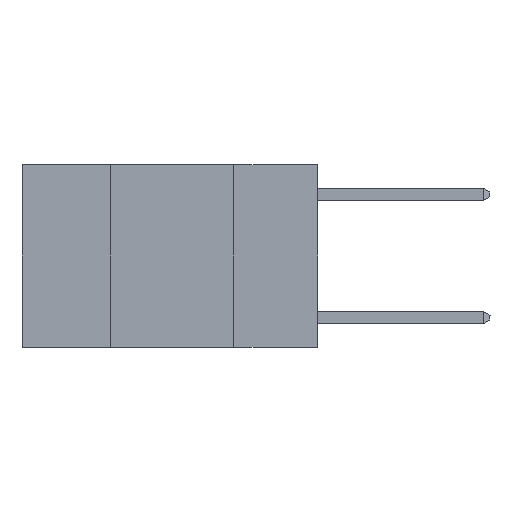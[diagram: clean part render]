
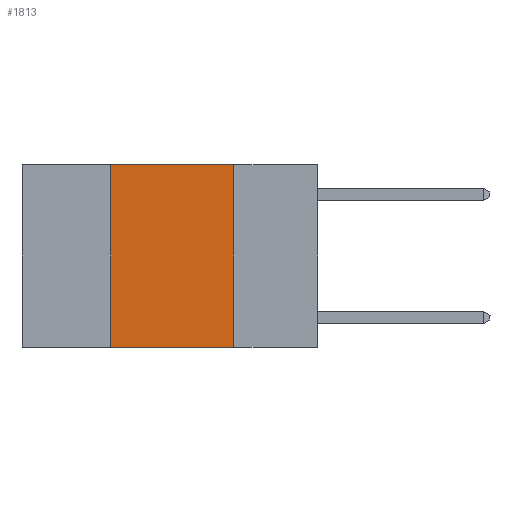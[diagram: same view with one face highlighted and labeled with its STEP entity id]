
A CAD part, left-side view. The second image highlights one B-rep face of the part: STEP entity #1813.
In plain terms, the highlighted planar face has unit normal (-1, 0, 0).
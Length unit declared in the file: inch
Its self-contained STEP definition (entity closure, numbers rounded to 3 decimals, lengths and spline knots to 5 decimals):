
#105 = CARTESIAN_POINT ( 'NONE',  ( 0., 0.6, 0. ) ) ;
#199 = EDGE_CURVE ( 'NONE', #4627, #4568, #7229, .T. ) ;
#1619 = DIRECTION ( 'NONE',  ( 0., -1., 0. ) ) ;
#1813 = ADVANCED_FACE ( 'NONE', ( #17642 ), #10746, .F. ) ;
#2471 = CARTESIAN_POINT ( 'NONE',  ( 0., 0.42, 0. ) ) ;
#3168 = DIRECTION ( 'NONE',  ( 0., -1., 0. ) ) ;
#3642 = DIRECTION ( 'NONE',  ( 0., 0., 1. ) ) ;
#4334 = CARTESIAN_POINT ( 'NONE',  ( 0., 0.42, -0.37 ) ) ;
#4423 = EDGE_CURVE ( 'NONE', #17658, #17810, #11080, .T. ) ;
#4512 = ORIENTED_EDGE ( 'NONE', *, *, #7670, .T. ) ;
#4556 = DIRECTION ( 'NONE',  ( 0., 0., -1. ) ) ;
#4568 = VERTEX_POINT ( 'NONE', #15377 ) ;
#4627 = VERTEX_POINT ( 'NONE', #8322 ) ;
#4974 = VECTOR ( 'NONE', #3642, 39.37008 ) ;
#5052 = DIRECTION ( 'NONE',  ( 0., 0., -1. ) ) ;
#5207 = ORIENTED_EDGE ( 'NONE', *, *, #199, .F. ) ;
#6779 = ORIENTED_EDGE ( 'NONE', *, *, #8624, .F. ) ;
#6850 = CARTESIAN_POINT ( 'NONE',  ( 0., 0.42, 0. ) ) ;
#7229 = LINE ( 'NONE', #10254, #7564 ) ;
#7535 = VECTOR ( 'NONE', #3168, 39.37008 ) ;
#7564 = VECTOR ( 'NONE', #4556, 39.37008 ) ;
#7670 = EDGE_CURVE ( 'NONE', #17658, #4568, #8884, .T. ) ;
#8236 = EDGE_LOOP ( 'NONE', ( #5207, #6779, #14369, #4512 ) ) ;
#8322 = CARTESIAN_POINT ( 'NONE',  ( 0., 0.17, 0. ) ) ;
#8599 = CARTESIAN_POINT ( 'NONE',  ( 0., 0.6, -0.37 ) ) ;
#8624 = EDGE_CURVE ( 'NONE', #17810, #4627, #16936, .T. ) ;
#8884 = LINE ( 'NONE', #8599, #14267 ) ;
#10254 = CARTESIAN_POINT ( 'NONE',  ( 0., 0.17, 0. ) ) ;
#10746 = PLANE ( 'NONE',  #10968 ) ;
#10968 = AXIS2_PLACEMENT_3D ( 'NONE', #13439, #14965, #5052 ) ;
#11080 = LINE ( 'NONE', #6850, #4974 ) ;
#13439 = CARTESIAN_POINT ( 'NONE',  ( 0., 0.6, 0. ) ) ;
#14267 = VECTOR ( 'NONE', #1619, 39.37008 ) ;
#14369 = ORIENTED_EDGE ( 'NONE', *, *, #4423, .F. ) ;
#14965 = DIRECTION ( 'NONE',  ( 1., 0., 0. ) ) ;
#15377 = CARTESIAN_POINT ( 'NONE',  ( 0., 0.17, -0.37 ) ) ;
#16936 = LINE ( 'NONE', #105, #7535 ) ;
#17642 = FACE_OUTER_BOUND ( 'NONE', #8236, .T. ) ;
#17658 = VERTEX_POINT ( 'NONE', #4334 ) ;
#17810 = VERTEX_POINT ( 'NONE', #2471 ) ;
